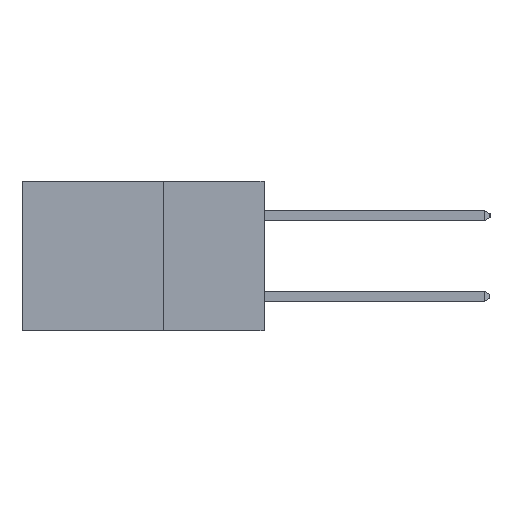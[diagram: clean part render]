
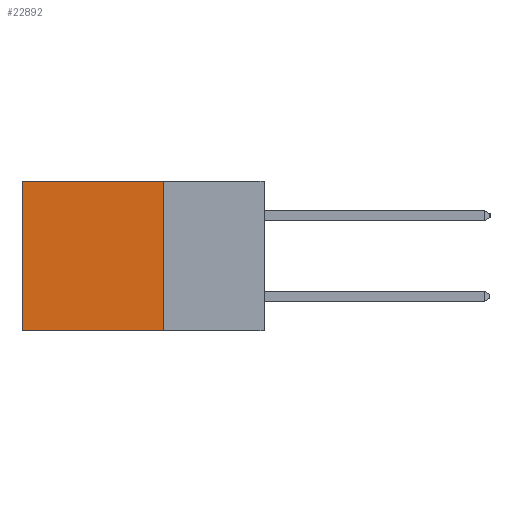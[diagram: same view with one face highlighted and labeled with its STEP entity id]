
A CAD part, left-side view. The second image highlights one B-rep face of the part: STEP entity #22892.
In plain terms, the highlighted planar face has unit normal (-1, 0, 0).
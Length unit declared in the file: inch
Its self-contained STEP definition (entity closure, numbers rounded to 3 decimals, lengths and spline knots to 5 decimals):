
#767 = VERTEX_POINT ( 'NONE', #9853 ) ;
#867 = EDGE_LOOP ( 'NONE', ( #11539, #26805, #26186, #2255 ) ) ;
#1135 = LINE ( 'NONE', #7034, #6450 ) ;
#1195 = LINE ( 'NONE', #26149, #24220 ) ;
#1494 = VERTEX_POINT ( 'NONE', #8968 ) ;
#2255 = ORIENTED_EDGE ( 'NONE', *, *, #20570, .T. ) ;
#4396 = AXIS2_PLACEMENT_3D ( 'NONE', #19531, #9121, #17488 ) ;
#6161 = CARTESIAN_POINT ( 'NONE',  ( 0.2615, 0.6, -0.37 ) ) ;
#6229 = DIRECTION ( 'NONE',  ( 0., 1., 0. ) ) ;
#6450 = VECTOR ( 'NONE', #11414, 39.37008 ) ;
#7034 = CARTESIAN_POINT ( 'NONE',  ( 0.2615, 0.25, 0. ) ) ;
#7273 = VERTEX_POINT ( 'NONE', #9253 ) ;
#8968 = CARTESIAN_POINT ( 'NONE',  ( 0.2615, 0.6, -0.37 ) ) ;
#9121 = DIRECTION ( 'NONE',  ( 1., 0., 0. ) ) ;
#9253 = CARTESIAN_POINT ( 'NONE',  ( 0.2615, 0.6, 0. ) ) ;
#9853 = CARTESIAN_POINT ( 'NONE',  ( 0.2615, 0.25, -0.37 ) ) ;
#9885 = DIRECTION ( 'NONE',  ( 0., 0., -1. ) ) ;
#11166 = FACE_OUTER_BOUND ( 'NONE', #867, .T. ) ;
#11414 = DIRECTION ( 'NONE',  ( 0., 1., 0. ) ) ;
#11539 = ORIENTED_EDGE ( 'NONE', *, *, #21116, .T. ) ;
#14322 = EDGE_CURVE ( 'NONE', #16008, #767, #1195, .T. ) ;
#16008 = VERTEX_POINT ( 'NONE', #21237 ) ;
#16336 = EDGE_CURVE ( 'NONE', #767, #1494, #25143, .T. ) ;
#17488 = DIRECTION ( 'NONE',  ( 0., 0., -1. ) ) ;
#18365 = LINE ( 'NONE', #6161, #27038 ) ;
#19484 = VECTOR ( 'NONE', #6229, 39.37008 ) ;
#19531 = CARTESIAN_POINT ( 'NONE',  ( 0.2615, 0.25, -0.37 ) ) ;
#20570 = EDGE_CURVE ( 'NONE', #16008, #7273, #1135, .T. ) ;
#21116 = EDGE_CURVE ( 'NONE', #7273, #1494, #18365, .T. ) ;
#21237 = CARTESIAN_POINT ( 'NONE',  ( 0.2615, 0.25, 0. ) ) ;
#22037 = DIRECTION ( 'NONE',  ( 0., 0., -1. ) ) ;
#22545 = CARTESIAN_POINT ( 'NONE',  ( 0.2615, 0.25, -0.37 ) ) ;
#22892 = ADVANCED_FACE ( 'NONE', ( #11166 ), #25827, .F. ) ;
#24220 = VECTOR ( 'NONE', #22037, 39.37008 ) ;
#25143 = LINE ( 'NONE', #22545, #19484 ) ;
#25827 = PLANE ( 'NONE',  #4396 ) ;
#26149 = CARTESIAN_POINT ( 'NONE',  ( 0.2615, 0.25, -0.37 ) ) ;
#26186 = ORIENTED_EDGE ( 'NONE', *, *, #14322, .F. ) ;
#26805 = ORIENTED_EDGE ( 'NONE', *, *, #16336, .F. ) ;
#27038 = VECTOR ( 'NONE', #9885, 39.37008 ) ;
